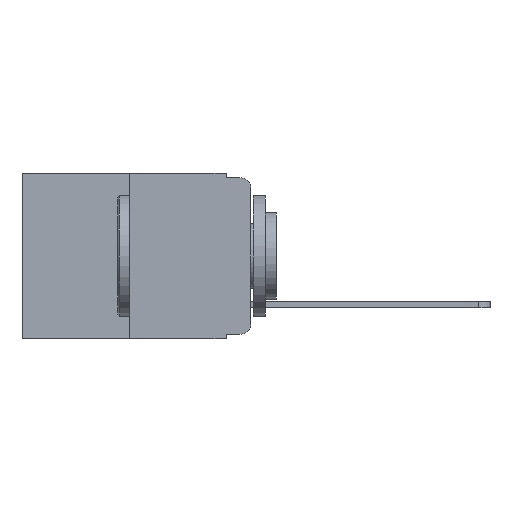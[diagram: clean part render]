
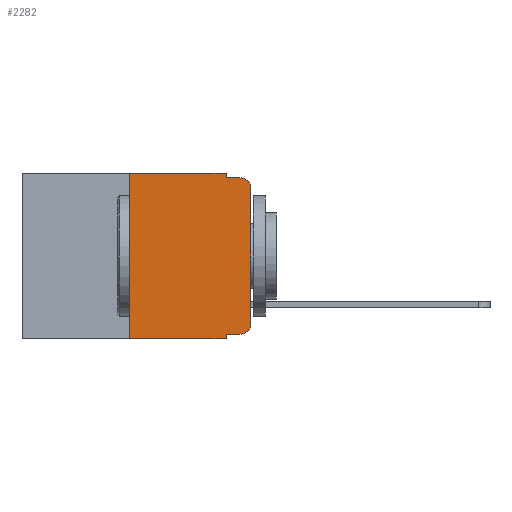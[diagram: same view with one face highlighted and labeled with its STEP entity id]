
A CAD part, left-side view. The second image highlights one B-rep face of the part: STEP entity #2282.
In plain terms, the highlighted planar face has unit normal (-1, 0, 0).
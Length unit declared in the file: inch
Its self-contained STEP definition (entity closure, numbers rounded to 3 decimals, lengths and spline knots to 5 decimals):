
#75 = VECTOR ( 'NONE', #151, 39.37008 ) ;
#151 = DIRECTION ( 'NONE',  ( 0., 0., 1. ) ) ;
#258 = AXIS2_PLACEMENT_3D ( 'NONE', #2131, #9381, #3217 ) ;
#440 = ORIENTED_EDGE ( 'NONE', *, *, #5440, .F. ) ;
#448 = CARTESIAN_POINT ( 'NONE',  ( 0., 0.051, -0.333 ) ) ;
#495 = CARTESIAN_POINT ( 'NONE',  ( 0., 0.051, -0.343 ) ) ;
#658 = VERTEX_POINT ( 'NONE', #3782 ) ;
#712 = CARTESIAN_POINT ( 'NONE',  ( 0., 0.051, -0.01 ) ) ;
#763 = ORIENTED_EDGE ( 'NONE', *, *, #6735, .T. ) ;
#1114 = LINE ( 'NONE', #9153, #6152 ) ;
#1221 = CARTESIAN_POINT ( 'NONE',  ( 0., 0.473, 0. ) ) ;
#1515 = CARTESIAN_POINT ( 'NONE',  ( 0., 0.02, -0.333 ) ) ;
#1786 = EDGE_CURVE ( 'NONE', #3105, #2697, #3161, .T. ) ;
#1899 = LINE ( 'NONE', #10018, #6901 ) ;
#2110 = AXIS2_PLACEMENT_3D ( 'NONE', #1221, #12409, #7692 ) ;
#2131 = CARTESIAN_POINT ( 'NONE',  ( 0., 0.02, -0.03 ) ) ;
#2282 = ADVANCED_FACE ( 'NONE', ( #8039 ), #7804, .F. ) ;
#2424 = EDGE_CURVE ( 'NONE', #8932, #8629, #1114, .T. ) ;
#2492 = EDGE_CURVE ( 'NONE', #3105, #8975, #13113, .T. ) ;
#2515 = CARTESIAN_POINT ( 'NONE',  ( 0., 0.051, -0.333 ) ) ;
#2697 = VERTEX_POINT ( 'NONE', #495 ) ;
#3099 = CARTESIAN_POINT ( 'NONE',  ( 0., 0.25, -0.343 ) ) ;
#3105 = VERTEX_POINT ( 'NONE', #2515 ) ;
#3156 = VECTOR ( 'NONE', #7108, 39.37008 ) ;
#3161 = LINE ( 'NONE', #9890, #6330 ) ;
#3217 = DIRECTION ( 'NONE',  ( 0., 0., -1. ) ) ;
#3293 = LINE ( 'NONE', #12482, #75 ) ;
#3362 = VERTEX_POINT ( 'NONE', #8970 ) ;
#3403 = VERTEX_POINT ( 'NONE', #3099 ) ;
#3490 = ORIENTED_EDGE ( 'NONE', *, *, #1786, .F. ) ;
#3535 = CARTESIAN_POINT ( 'NONE',  ( 0., 0.02, -0.313 ) ) ;
#3648 = CARTESIAN_POINT ( 'NONE',  ( 0., 0., -0.313 ) ) ;
#3782 = CARTESIAN_POINT ( 'NONE',  ( 0., 0.25, 0. ) ) ;
#3857 = LINE ( 'NONE', #6047, #3156 ) ;
#4017 = ORIENTED_EDGE ( 'NONE', *, *, #2492, .T. ) ;
#4352 = ORIENTED_EDGE ( 'NONE', *, *, #2424, .T. ) ;
#4638 = DIRECTION ( 'NONE',  ( 0., 0., -1. ) ) ;
#4764 = CARTESIAN_POINT ( 'NONE',  ( 0., 0.051, 0. ) ) ;
#4820 = ORIENTED_EDGE ( 'NONE', *, *, #12917, .T. ) ;
#4910 = VECTOR ( 'NONE', #5798, 39.37008 ) ;
#5007 = DIRECTION ( 'NONE',  ( 0., -1., 0. ) ) ;
#5139 = VERTEX_POINT ( 'NONE', #712 ) ;
#5188 = VECTOR ( 'NONE', #12977, 39.37008 ) ;
#5377 = ORIENTED_EDGE ( 'NONE', *, *, #10361, .T. ) ;
#5440 = EDGE_CURVE ( 'NONE', #3403, #658, #3293, .T. ) ;
#5655 = ORIENTED_EDGE ( 'NONE', *, *, #12264, .F. ) ;
#5798 = DIRECTION ( 'NONE',  ( 0., 0., -1. ) ) ;
#6047 = CARTESIAN_POINT ( 'NONE',  ( 0., 0.051, -0.01 ) ) ;
#6152 = VECTOR ( 'NONE', #8544, 39.37008 ) ;
#6161 = CIRCLE ( 'NONE', #8196, 0.02 ) ;
#6330 = VECTOR ( 'NONE', #8711, 39.37008 ) ;
#6335 = CARTESIAN_POINT ( 'NONE',  ( 0., 0., -0.03 ) ) ;
#6613 = EDGE_LOOP ( 'NONE', ( #4352, #4820, #5655, #7028, #8024, #440, #763, #3490, #4017, #5377 ) ) ;
#6735 = EDGE_CURVE ( 'NONE', #3403, #2697, #1899, .T. ) ;
#6901 = VECTOR ( 'NONE', #5007, 39.37008 ) ;
#7028 = ORIENTED_EDGE ( 'NONE', *, *, #8951, .F. ) ;
#7108 = DIRECTION ( 'NONE',  ( 0., -1., 0. ) ) ;
#7498 = DIRECTION ( 'NONE',  ( 0., -1., 0. ) ) ;
#7612 = LINE ( 'NONE', #4764, #4910 ) ;
#7692 = DIRECTION ( 'NONE',  ( 0., 0., -1. ) ) ;
#7754 = VECTOR ( 'NONE', #7498, 39.37008 ) ;
#7804 = PLANE ( 'NONE',  #2110 ) ;
#8024 = ORIENTED_EDGE ( 'NONE', *, *, #11830, .F. ) ;
#8039 = FACE_OUTER_BOUND ( 'NONE', #6613, .T. ) ;
#8196 = AXIS2_PLACEMENT_3D ( 'NONE', #3535, #10650, #4638 ) ;
#8544 = DIRECTION ( 'NONE',  ( 0., 0., 1. ) ) ;
#8629 = VERTEX_POINT ( 'NONE', #6335 ) ;
#8711 = DIRECTION ( 'NONE',  ( 0., 0., -1. ) ) ;
#8932 = VERTEX_POINT ( 'NONE', #3648 ) ;
#8951 = EDGE_CURVE ( 'NONE', #10651, #5139, #7612, .T. ) ;
#8970 = CARTESIAN_POINT ( 'NONE',  ( 0., 0.02, -0.01 ) ) ;
#8975 = VERTEX_POINT ( 'NONE', #1515 ) ;
#9153 = CARTESIAN_POINT ( 'NONE',  ( 0., 0., 0. ) ) ;
#9381 = DIRECTION ( 'NONE',  ( -1., 0., 0. ) ) ;
#9493 = CARTESIAN_POINT ( 'NONE',  ( 0., 0.473, 0. ) ) ;
#9890 = CARTESIAN_POINT ( 'NONE',  ( 0., 0.051, 0. ) ) ;
#10018 = CARTESIAN_POINT ( 'NONE',  ( 0., 0.473, -0.343 ) ) ;
#10361 = EDGE_CURVE ( 'NONE', #8975, #8932, #6161, .T. ) ;
#10650 = DIRECTION ( 'NONE',  ( -1., 0., 0. ) ) ;
#10651 = VERTEX_POINT ( 'NONE', #11890 ) ;
#10811 = CIRCLE ( 'NONE', #258, 0.02 ) ;
#11830 = EDGE_CURVE ( 'NONE', #658, #10651, #12990, .T. ) ;
#11890 = CARTESIAN_POINT ( 'NONE',  ( 0., 0.051, 0. ) ) ;
#12264 = EDGE_CURVE ( 'NONE', #5139, #3362, #3857, .T. ) ;
#12409 = DIRECTION ( 'NONE',  ( 1., 0., 0. ) ) ;
#12482 = CARTESIAN_POINT ( 'NONE',  ( 0., 0.25, 0. ) ) ;
#12917 = EDGE_CURVE ( 'NONE', #8629, #3362, #10811, .T. ) ;
#12977 = DIRECTION ( 'NONE',  ( 0., -1., 0. ) ) ;
#12990 = LINE ( 'NONE', #9493, #7754 ) ;
#13113 = LINE ( 'NONE', #448, #5188 ) ;
